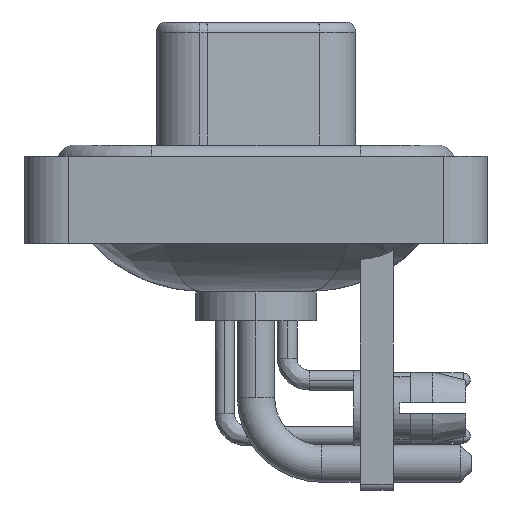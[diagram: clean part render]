
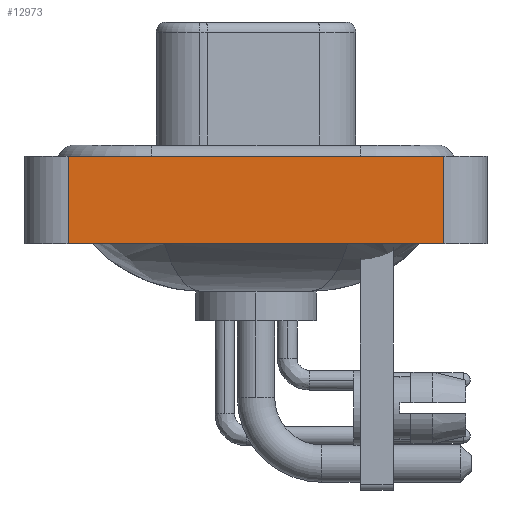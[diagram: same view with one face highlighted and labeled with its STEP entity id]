
A CAD part, left-side view. The second image highlights one B-rep face of the part: STEP entity #12973.
In plain terms, the highlighted planar face has unit normal (-1, 0, 0).
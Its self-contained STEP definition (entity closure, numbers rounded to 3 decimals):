
#278 = DIRECTION ( 'NONE',  ( 0., -1., 0. ) ) ;
#377 = LINE ( 'NONE', #9923, #14120 ) ;
#1539 = LINE ( 'NONE', #30065, #4892 ) ;
#1830 = ORIENTED_EDGE ( 'NONE', *, *, #22013, .F. ) ;
#2204 = ORIENTED_EDGE ( 'NONE', *, *, #13572, .T. ) ;
#2935 = VERTEX_POINT ( 'NONE', #5945 ) ;
#3490 = LINE ( 'NONE', #25337, #26124 ) ;
#4849 = EDGE_LOOP ( 'NONE', ( #28988, #17989, #1830, #2204 ) ) ;
#4892 = VECTOR ( 'NONE', #28197, 1000. ) ;
#5945 = CARTESIAN_POINT ( 'NONE',  ( -7.35, -8.55, 0.4 ) ) ;
#9923 = CARTESIAN_POINT ( 'NONE',  ( -7.35, -8.55, 0.4 ) ) ;
#10068 = DIRECTION ( 'NONE',  ( 0., -1., 0. ) ) ;
#11406 = CARTESIAN_POINT ( 'NONE',  ( -7.35, -8.55, -3.6 ) ) ;
#12973 = ADVANCED_FACE ( 'NONE', ( #20017 ), #12998, .T. ) ;
#12998 = PLANE ( 'NONE',  #29564 ) ;
#13476 = VERTEX_POINT ( 'NONE', #11406 ) ;
#13572 = EDGE_CURVE ( 'NONE', #23489, #13476, #28494, .T. ) ;
#13852 = EDGE_CURVE ( 'NONE', #23697, #2935, #377, .T. ) ;
#14120 = VECTOR ( 'NONE', #10068, 1000. ) ;
#16278 = CARTESIAN_POINT ( 'NONE',  ( -7.35, 8.55, -3.6 ) ) ;
#17685 = CARTESIAN_POINT ( 'NONE',  ( -7.35, -8.55, -3.6 ) ) ;
#17989 = ORIENTED_EDGE ( 'NONE', *, *, #13852, .F. ) ;
#18922 = EDGE_CURVE ( 'NONE', #13476, #2935, #1539, .T. ) ;
#19235 = CARTESIAN_POINT ( 'NONE',  ( -7.35, 8.55, 0.4 ) ) ;
#19344 = CARTESIAN_POINT ( 'NONE',  ( -7.35, -8.55, -3.6 ) ) ;
#20017 = FACE_OUTER_BOUND ( 'NONE', #4849, .T. ) ;
#22013 = EDGE_CURVE ( 'NONE', #23489, #23697, #3490, .T. ) ;
#22673 = DIRECTION ( 'NONE',  ( -1., 0., 0. ) ) ;
#23489 = VERTEX_POINT ( 'NONE', #16278 ) ;
#23697 = VERTEX_POINT ( 'NONE', #19235 ) ;
#24857 = DIRECTION ( 'NONE',  ( 0., 0., 1. ) ) ;
#25337 = CARTESIAN_POINT ( 'NONE',  ( -7.35, 8.55, -3.6 ) ) ;
#26124 = VECTOR ( 'NONE', #24857, 1000. ) ;
#27475 = DIRECTION ( 'NONE',  ( 0., 0., 1. ) ) ;
#27707 = VECTOR ( 'NONE', #278, 1000. ) ;
#28197 = DIRECTION ( 'NONE',  ( 0., 0., 1. ) ) ;
#28494 = LINE ( 'NONE', #19344, #27707 ) ;
#28988 = ORIENTED_EDGE ( 'NONE', *, *, #18922, .T. ) ;
#29564 = AXIS2_PLACEMENT_3D ( 'NONE', #17685, #22673, #27475 ) ;
#30065 = CARTESIAN_POINT ( 'NONE',  ( -7.35, -8.55, -3.6 ) ) ;
